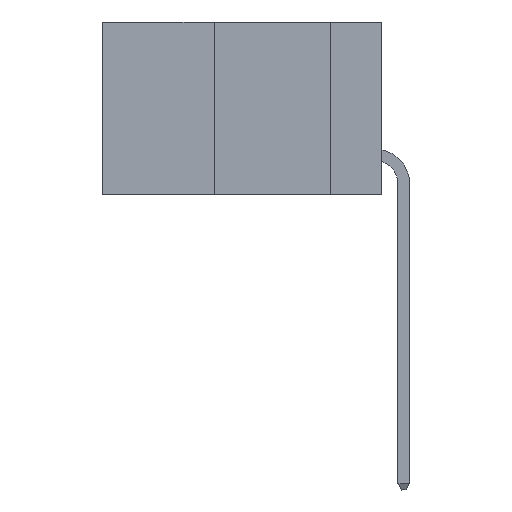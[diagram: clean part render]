
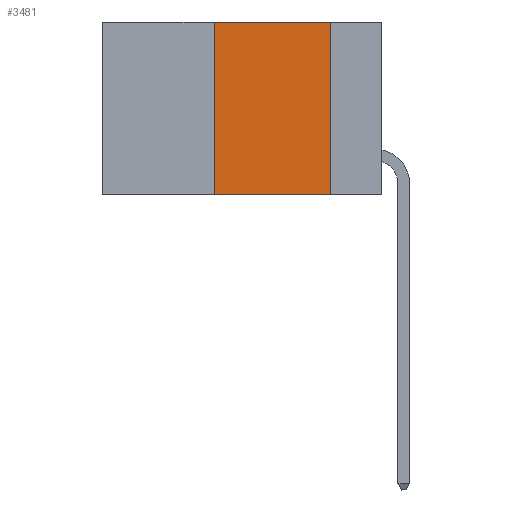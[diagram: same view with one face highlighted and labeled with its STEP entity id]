
A CAD part, left-side view. The second image highlights one B-rep face of the part: STEP entity #3481.
In plain terms, the highlighted planar face has unit normal (-1, 0, 0).
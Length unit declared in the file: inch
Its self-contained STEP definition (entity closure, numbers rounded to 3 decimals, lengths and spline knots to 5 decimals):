
#343 = DIRECTION ( 'NONE',  ( 1., 0., 0. ) ) ;
#512 = EDGE_CURVE ( 'NONE', #3296, #4470, #942, .T. ) ;
#942 = LINE ( 'NONE', #15601, #12424 ) ;
#1042 = EDGE_CURVE ( 'NONE', #4470, #8437, #1629, .T. ) ;
#1629 = LINE ( 'NONE', #6735, #8215 ) ;
#1769 = PLANE ( 'NONE',  #1891 ) ;
#1891 = AXIS2_PLACEMENT_3D ( 'NONE', #18281, #343, #2282 ) ;
#1981 = CARTESIAN_POINT ( 'NONE',  ( 0., 0.36, -0.37 ) ) ;
#2282 = DIRECTION ( 'NONE',  ( 0., 0., -1. ) ) ;
#3296 = VERTEX_POINT ( 'NONE', #12565 ) ;
#3481 = ADVANCED_FACE ( 'NONE', ( #12617 ), #1769, .F. ) ;
#3742 = DIRECTION ( 'NONE',  ( 0., -1., 0. ) ) ;
#4470 = VERTEX_POINT ( 'NONE', #9858 ) ;
#6067 = ORIENTED_EDGE ( 'NONE', *, *, #17910, .F. ) ;
#6074 = DIRECTION ( 'NONE',  ( 0., 0., 1. ) ) ;
#6735 = CARTESIAN_POINT ( 'NONE',  ( 0., 0.11, 0. ) ) ;
#6874 = DIRECTION ( 'NONE',  ( 0., -1., 0. ) ) ;
#7348 = ORIENTED_EDGE ( 'NONE', *, *, #512, .F. ) ;
#8215 = VECTOR ( 'NONE', #12196, 39.37008 ) ;
#8437 = VERTEX_POINT ( 'NONE', #13712 ) ;
#8848 = EDGE_LOOP ( 'NONE', ( #18070, #7348, #6067, #18347 ) ) ;
#9531 = VECTOR ( 'NONE', #6074, 39.37008 ) ;
#9858 = CARTESIAN_POINT ( 'NONE',  ( 0., 0.11, 0. ) ) ;
#10627 = CARTESIAN_POINT ( 'NONE',  ( 0., 0.36, 0. ) ) ;
#11819 = VECTOR ( 'NONE', #6874, 39.37008 ) ;
#12196 = DIRECTION ( 'NONE',  ( 0., 0., -1. ) ) ;
#12424 = VECTOR ( 'NONE', #3742, 39.37008 ) ;
#12565 = CARTESIAN_POINT ( 'NONE',  ( 0., 0.36, 0. ) ) ;
#12617 = FACE_OUTER_BOUND ( 'NONE', #8848, .T. ) ;
#13712 = CARTESIAN_POINT ( 'NONE',  ( 0., 0.11, -0.37 ) ) ;
#13731 = LINE ( 'NONE', #15866, #11819 ) ;
#13788 = LINE ( 'NONE', #10627, #9531 ) ;
#14861 = VERTEX_POINT ( 'NONE', #1981 ) ;
#15601 = CARTESIAN_POINT ( 'NONE',  ( 0., 0.6, 0. ) ) ;
#15866 = CARTESIAN_POINT ( 'NONE',  ( 0., 0.6, -0.37 ) ) ;
#17910 = EDGE_CURVE ( 'NONE', #14861, #3296, #13788, .T. ) ;
#18070 = ORIENTED_EDGE ( 'NONE', *, *, #1042, .F. ) ;
#18281 = CARTESIAN_POINT ( 'NONE',  ( 0., 0.6, 0. ) ) ;
#18347 = ORIENTED_EDGE ( 'NONE', *, *, #19162, .T. ) ;
#19162 = EDGE_CURVE ( 'NONE', #14861, #8437, #13731, .T. ) ;
